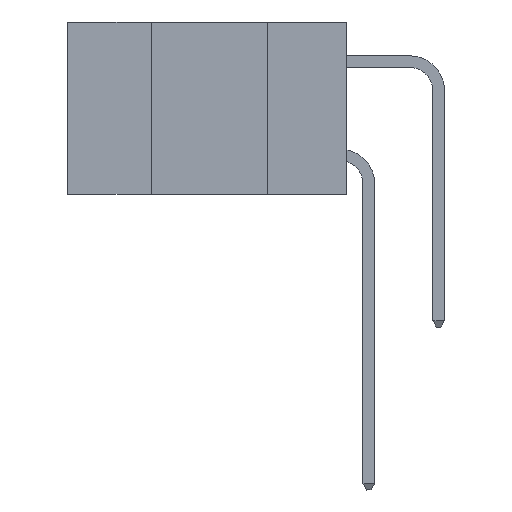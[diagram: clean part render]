
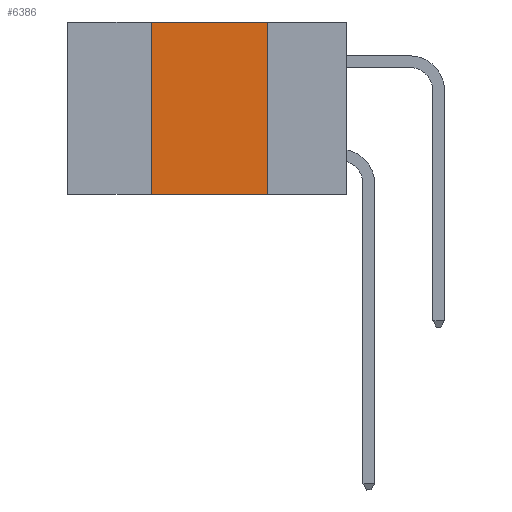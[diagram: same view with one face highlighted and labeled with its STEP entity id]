
A CAD part, left-side view. The second image highlights one B-rep face of the part: STEP entity #6386.
In plain terms, the highlighted planar face has unit normal (-1, 0, 0).
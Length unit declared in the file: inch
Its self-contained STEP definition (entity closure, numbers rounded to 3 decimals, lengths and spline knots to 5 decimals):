
#586 = ORIENTED_EDGE ( 'NONE', *, *, #7205, .F. ) ;
#828 = CARTESIAN_POINT ( 'NONE',  ( 0., 0.17, 0. ) ) ;
#1470 = CARTESIAN_POINT ( 'NONE',  ( 0., 0.6, 0. ) ) ;
#1744 = VECTOR ( 'NONE', #2027, 39.37008 ) ;
#1752 = ORIENTED_EDGE ( 'NONE', *, *, #7778, .F. ) ;
#1938 = DIRECTION ( 'NONE',  ( 0., 0., 1. ) ) ;
#2027 = DIRECTION ( 'NONE',  ( 0., 0., -1. ) ) ;
#2498 = VECTOR ( 'NONE', #5711, 39.37008 ) ;
#2530 = FACE_OUTER_BOUND ( 'NONE', #13273, .T. ) ;
#3733 = VERTEX_POINT ( 'NONE', #7905 ) ;
#3823 = EDGE_CURVE ( 'NONE', #9399, #12806, #11807, .T. ) ;
#4535 = CARTESIAN_POINT ( 'NONE',  ( 0., 0.6, -0.37 ) ) ;
#4737 = DIRECTION ( 'NONE',  ( 0., -1., 0. ) ) ;
#5711 = DIRECTION ( 'NONE',  ( 0., -1., 0. ) ) ;
#6386 = ADVANCED_FACE ( 'NONE', ( #2530 ), #14337, .F. ) ;
#7205 = EDGE_CURVE ( 'NONE', #3733, #9399, #13990, .T. ) ;
#7230 = VECTOR ( 'NONE', #4737, 39.37008 ) ;
#7509 = CARTESIAN_POINT ( 'NONE',  ( 0., 0.17, 0. ) ) ;
#7778 = EDGE_CURVE ( 'NONE', #12806, #12985, #11621, .T. ) ;
#7905 = CARTESIAN_POINT ( 'NONE',  ( 0., 0.42, -0.37 ) ) ;
#8816 = ORIENTED_EDGE ( 'NONE', *, *, #3823, .F. ) ;
#9376 = CARTESIAN_POINT ( 'NONE',  ( 0., 0.17, -0.37 ) ) ;
#9399 = VERTEX_POINT ( 'NONE', #9912 ) ;
#9912 = CARTESIAN_POINT ( 'NONE',  ( 0., 0.42, 0. ) ) ;
#10984 = DIRECTION ( 'NONE',  ( 1., 0., 0. ) ) ;
#11275 = VECTOR ( 'NONE', #1938, 39.37008 ) ;
#11621 = LINE ( 'NONE', #828, #1744 ) ;
#11807 = LINE ( 'NONE', #15106, #2498 ) ;
#12089 = ORIENTED_EDGE ( 'NONE', *, *, #13955, .T. ) ;
#12806 = VERTEX_POINT ( 'NONE', #7509 ) ;
#12985 = VERTEX_POINT ( 'NONE', #9376 ) ;
#13126 = LINE ( 'NONE', #4535, #7230 ) ;
#13273 = EDGE_LOOP ( 'NONE', ( #1752, #8816, #586, #12089 ) ) ;
#13498 = CARTESIAN_POINT ( 'NONE',  ( 0., 0.42, 0. ) ) ;
#13955 = EDGE_CURVE ( 'NONE', #3733, #12985, #13126, .T. ) ;
#13990 = LINE ( 'NONE', #13498, #11275 ) ;
#14178 = AXIS2_PLACEMENT_3D ( 'NONE', #1470, #10984, #14232 ) ;
#14232 = DIRECTION ( 'NONE',  ( 0., 0., -1. ) ) ;
#14337 = PLANE ( 'NONE',  #14178 ) ;
#15106 = CARTESIAN_POINT ( 'NONE',  ( 0., 0.6, 0. ) ) ;
